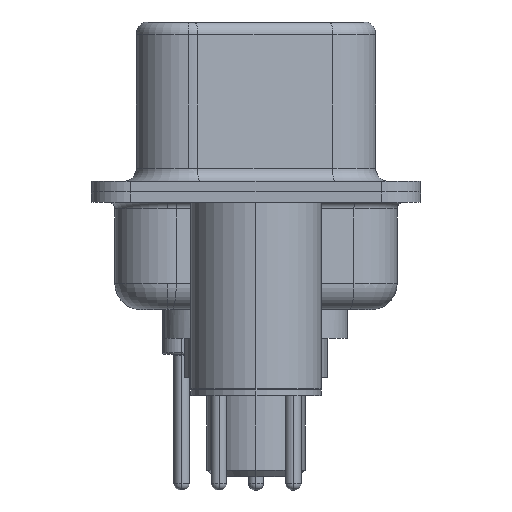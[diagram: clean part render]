
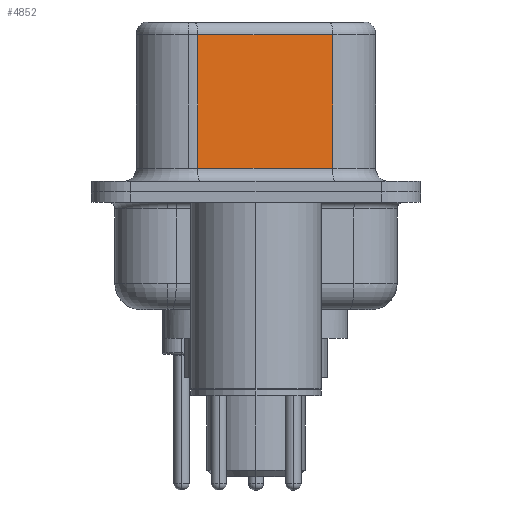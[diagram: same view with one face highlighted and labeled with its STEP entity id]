
A CAD part, left-side view. The second image highlights one B-rep face of the part: STEP entity #4852.
In plain terms, the highlighted planar face has unit normal (-0.985, -0.174, 0).
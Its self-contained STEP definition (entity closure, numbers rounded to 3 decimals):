
#2424 = EDGE_CURVE ( 'NONE', #14130, #2499, #18433, .T. ) ;
#2499 = VERTEX_POINT ( 'NONE', #19115 ) ;
#2646 = FACE_OUTER_BOUND ( 'NONE', #16245, .T. ) ;
#3809 = DIRECTION ( 'NONE',  ( 0., 0., -1. ) ) ;
#4785 = VERTEX_POINT ( 'NONE', #5619 ) ;
#4852 = ADVANCED_FACE ( 'NONE', ( #2646 ), #14419, .F. ) ;
#5573 = EDGE_CURVE ( 'NONE', #12876, #4785, #17011, .T. ) ;
#5619 = CARTESIAN_POINT ( 'NONE',  ( 4.585, -2.927, 0.9 ) ) ;
#6111 = DIRECTION ( 'NONE',  ( -0.174, 0.985, 0. ) ) ;
#6955 = EDGE_CURVE ( 'NONE', #12876, #14130, #8259, .T. ) ;
#7257 = VECTOR ( 'NONE', #3809, 1000. ) ;
#7823 = LINE ( 'NONE', #20325, #12452 ) ;
#8259 = LINE ( 'NONE', #10049, #19046 ) ;
#8473 = DIRECTION ( 'NONE',  ( -0.174, 0.985, 0. ) ) ;
#9377 = DIRECTION ( 'NONE',  ( 0.985, 0.174, 0. ) ) ;
#9672 = VECTOR ( 'NONE', #17607, 1000. ) ;
#10001 = EDGE_CURVE ( 'NONE', #2499, #4785, #7823, .T. ) ;
#10049 = CARTESIAN_POINT ( 'NONE',  ( 4.585, -2.927, 6.02 ) ) ;
#10934 = CARTESIAN_POINT ( 'NONE',  ( 3.675, 2.233, 6.02 ) ) ;
#11195 = CARTESIAN_POINT ( 'NONE',  ( 4.585, -2.927, 6.52 ) ) ;
#11873 = CARTESIAN_POINT ( 'NONE',  ( 4.585, -2.927, 6.02 ) ) ;
#12452 = VECTOR ( 'NONE', #13392, 1000. ) ;
#12507 = CARTESIAN_POINT ( 'NONE',  ( 3.675, 2.233, 6.52 ) ) ;
#12621 = ORIENTED_EDGE ( 'NONE', *, *, #5573, .F. ) ;
#12876 = VERTEX_POINT ( 'NONE', #11873 ) ;
#13392 = DIRECTION ( 'NONE',  ( 0.174, -0.985, 0. ) ) ;
#13532 = AXIS2_PLACEMENT_3D ( 'NONE', #11195, #9377, #6111 ) ;
#14130 = VERTEX_POINT ( 'NONE', #10934 ) ;
#14419 = PLANE ( 'NONE',  #13532 ) ;
#16245 = EDGE_LOOP ( 'NONE', ( #12621, #18355, #17723, #16721 ) ) ;
#16721 = ORIENTED_EDGE ( 'NONE', *, *, #10001, .T. ) ;
#17011 = LINE ( 'NONE', #18511, #7257 ) ;
#17607 = DIRECTION ( 'NONE',  ( 0., 0., -1. ) ) ;
#17723 = ORIENTED_EDGE ( 'NONE', *, *, #2424, .T. ) ;
#18355 = ORIENTED_EDGE ( 'NONE', *, *, #6955, .T. ) ;
#18433 = LINE ( 'NONE', #12507, #9672 ) ;
#18511 = CARTESIAN_POINT ( 'NONE',  ( 4.585, -2.927, 6.52 ) ) ;
#19046 = VECTOR ( 'NONE', #8473, 1000. ) ;
#19115 = CARTESIAN_POINT ( 'NONE',  ( 3.675, 2.233, 0.9 ) ) ;
#20325 = CARTESIAN_POINT ( 'NONE',  ( 4.585, -2.927, 0.9 ) ) ;
